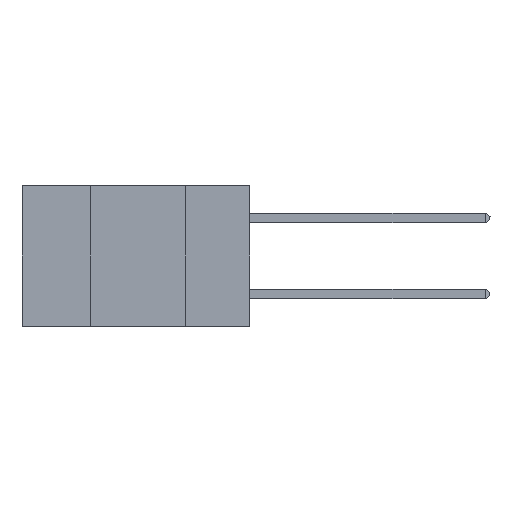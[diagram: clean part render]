
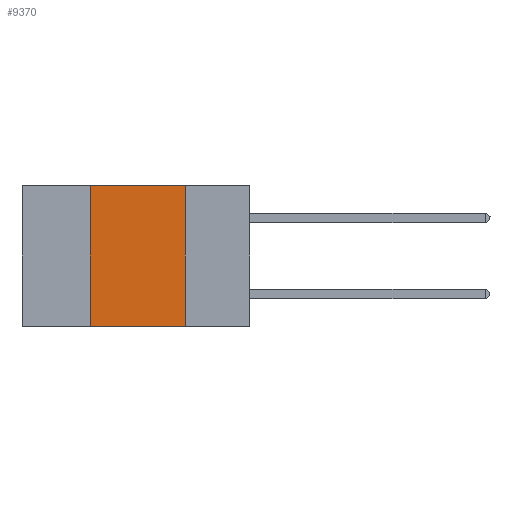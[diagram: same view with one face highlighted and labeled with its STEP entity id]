
A CAD part, left-side view. The second image highlights one B-rep face of the part: STEP entity #9370.
In plain terms, the highlighted planar face has unit normal (-1, 0, 0).
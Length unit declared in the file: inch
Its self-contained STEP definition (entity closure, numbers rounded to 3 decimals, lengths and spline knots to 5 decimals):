
#575 = EDGE_CURVE ( 'NONE', #39818, #12611, #12662, .T. ) ;
#3326 = DIRECTION ( 'NONE',  ( 0., 0., -1. ) ) ;
#9048 = VERTEX_POINT ( 'NONE', #36337 ) ;
#9370 = ADVANCED_FACE ( 'NONE', ( #18863 ), #41835, .F. ) ;
#9729 = DIRECTION ( 'NONE',  ( 0., 0., -1. ) ) ;
#10844 = VECTOR ( 'NONE', #22124, 39.37008 ) ;
#12611 = VERTEX_POINT ( 'NONE', #35625 ) ;
#12662 = LINE ( 'NONE', #37820, #18384 ) ;
#13838 = VECTOR ( 'NONE', #3326, 39.37008 ) ;
#15151 = CARTESIAN_POINT ( 'NONE',  ( 0., 0.42, 0. ) ) ;
#15846 = AXIS2_PLACEMENT_3D ( 'NONE', #31841, #38859, #9729 ) ;
#18384 = VECTOR ( 'NONE', #32222, 39.37008 ) ;
#18863 = FACE_OUTER_BOUND ( 'NONE', #19827, .T. ) ;
#19827 = EDGE_LOOP ( 'NONE', ( #33210, #35794, #23548, #31481 ) ) ;
#22124 = DIRECTION ( 'NONE',  ( 0., -1., 0. ) ) ;
#22887 = LINE ( 'NONE', #39261, #13838 ) ;
#23122 = EDGE_CURVE ( 'NONE', #39818, #31507, #35115, .T. ) ;
#23548 = ORIENTED_EDGE ( 'NONE', *, *, #23122, .F. ) ;
#25122 = LINE ( 'NONE', #35106, #10844 ) ;
#25349 = DIRECTION ( 'NONE',  ( 0., 0., 1. ) ) ;
#25884 = EDGE_CURVE ( 'NONE', #31507, #9048, #25122, .T. ) ;
#29252 = VECTOR ( 'NONE', #25349, 39.37008 ) ;
#31481 = ORIENTED_EDGE ( 'NONE', *, *, #575, .T. ) ;
#31507 = VERTEX_POINT ( 'NONE', #15151 ) ;
#31841 = CARTESIAN_POINT ( 'NONE',  ( 0., 0.6, 0. ) ) ;
#32138 = CARTESIAN_POINT ( 'NONE',  ( 0., 0.42, 0. ) ) ;
#32222 = DIRECTION ( 'NONE',  ( 0., -1., 0. ) ) ;
#33210 = ORIENTED_EDGE ( 'NONE', *, *, #36728, .F. ) ;
#35106 = CARTESIAN_POINT ( 'NONE',  ( 0., 0.6, 0. ) ) ;
#35115 = LINE ( 'NONE', #32138, #29252 ) ;
#35625 = CARTESIAN_POINT ( 'NONE',  ( 0., 0.17, -0.37 ) ) ;
#35794 = ORIENTED_EDGE ( 'NONE', *, *, #25884, .F. ) ;
#36337 = CARTESIAN_POINT ( 'NONE',  ( 0., 0.17, 0. ) ) ;
#36728 = EDGE_CURVE ( 'NONE', #9048, #12611, #22887, .T. ) ;
#37820 = CARTESIAN_POINT ( 'NONE',  ( 0., 0.6, -0.37 ) ) ;
#38245 = CARTESIAN_POINT ( 'NONE',  ( 0., 0.42, -0.37 ) ) ;
#38859 = DIRECTION ( 'NONE',  ( 1., 0., 0. ) ) ;
#39261 = CARTESIAN_POINT ( 'NONE',  ( 0., 0.17, 0. ) ) ;
#39818 = VERTEX_POINT ( 'NONE', #38245 ) ;
#41835 = PLANE ( 'NONE',  #15846 ) ;
